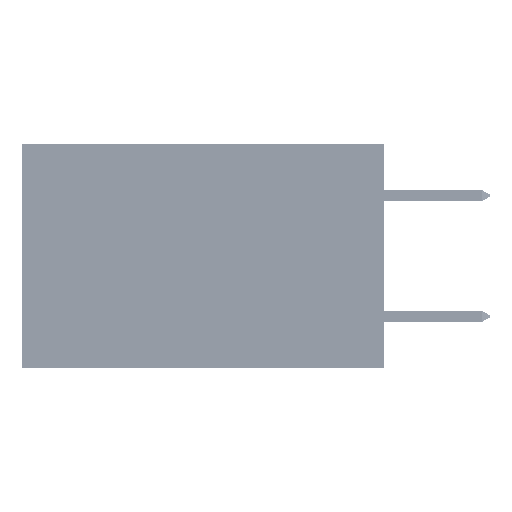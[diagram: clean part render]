
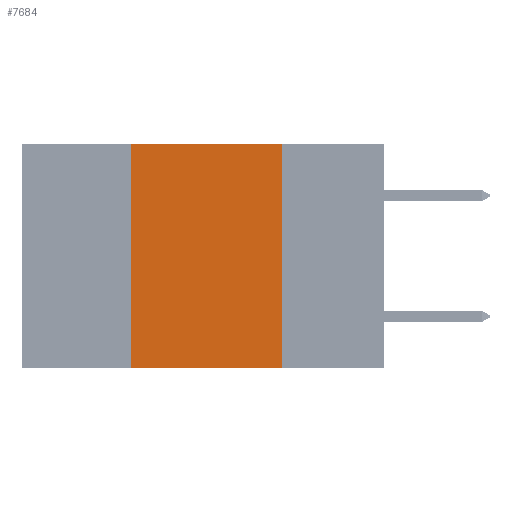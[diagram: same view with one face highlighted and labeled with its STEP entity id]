
A CAD part, left-side view. The second image highlights one B-rep face of the part: STEP entity #7684.
In plain terms, the highlighted planar face has unit normal (-1, 0, 0).
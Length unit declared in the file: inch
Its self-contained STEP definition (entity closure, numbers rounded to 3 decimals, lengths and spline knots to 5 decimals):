
#2695 = EDGE_LOOP ( 'NONE', ( #38751, #36651, #32935, #32762 ) ) ;
#6746 = EDGE_CURVE ( 'NONE', #7051, #33183, #30985, .T. ) ;
#7051 = VERTEX_POINT ( 'NONE', #43044 ) ;
#7213 = CARTESIAN_POINT ( 'NONE',  ( 0., 0.17, -0.37 ) ) ;
#7396 = VERTEX_POINT ( 'NONE', #7213 ) ;
#7684 = ADVANCED_FACE ( 'NONE', ( #33970 ), #12927, .F. ) ;
#9868 = VECTOR ( 'NONE', #33888, 39.37008 ) ;
#10032 = VECTOR ( 'NONE', #12802, 39.37008 ) ;
#12802 = DIRECTION ( 'NONE',  ( 0., 0., -1. ) ) ;
#12927 = PLANE ( 'NONE',  #21436 ) ;
#16139 = CARTESIAN_POINT ( 'NONE',  ( 0., 0.17, 0. ) ) ;
#16588 = DIRECTION ( 'NONE',  ( 0., 0., -1. ) ) ;
#20619 = LINE ( 'NONE', #16139, #10032 ) ;
#21436 = AXIS2_PLACEMENT_3D ( 'NONE', #40287, #24396, #16588 ) ;
#21465 = CARTESIAN_POINT ( 'NONE',  ( 0., 0.17, 0. ) ) ;
#21506 = EDGE_CURVE ( 'NONE', #43716, #7396, #25130, .T. ) ;
#24396 = DIRECTION ( 'NONE',  ( 1., 0., 0. ) ) ;
#25130 = LINE ( 'NONE', #29397, #26310 ) ;
#25636 = LINE ( 'NONE', #34599, #39239 ) ;
#26310 = VECTOR ( 'NONE', #29555, 39.37008 ) ;
#29397 = CARTESIAN_POINT ( 'NONE',  ( 0., 0.6, -0.37 ) ) ;
#29547 = CARTESIAN_POINT ( 'NONE',  ( 0., 0.6, 0. ) ) ;
#29555 = DIRECTION ( 'NONE',  ( 0., -1., 0. ) ) ;
#30985 = LINE ( 'NONE', #29547, #9868 ) ;
#32762 = ORIENTED_EDGE ( 'NONE', *, *, #21506, .T. ) ;
#32935 = ORIENTED_EDGE ( 'NONE', *, *, #47032, .F. ) ;
#33183 = VERTEX_POINT ( 'NONE', #21465 ) ;
#33888 = DIRECTION ( 'NONE',  ( 0., -1., 0. ) ) ;
#33970 = FACE_OUTER_BOUND ( 'NONE', #2695, .T. ) ;
#34599 = CARTESIAN_POINT ( 'NONE',  ( 0., 0.42, 0. ) ) ;
#34834 = CARTESIAN_POINT ( 'NONE',  ( 0., 0.42, -0.37 ) ) ;
#36651 = ORIENTED_EDGE ( 'NONE', *, *, #6746, .F. ) ;
#38751 = ORIENTED_EDGE ( 'NONE', *, *, #48564, .F. ) ;
#39239 = VECTOR ( 'NONE', #50597, 39.37008 ) ;
#40287 = CARTESIAN_POINT ( 'NONE',  ( 0., 0.6, 0. ) ) ;
#43044 = CARTESIAN_POINT ( 'NONE',  ( 0., 0.42, 0. ) ) ;
#43716 = VERTEX_POINT ( 'NONE', #34834 ) ;
#47032 = EDGE_CURVE ( 'NONE', #43716, #7051, #25636, .T. ) ;
#48564 = EDGE_CURVE ( 'NONE', #33183, #7396, #20619, .T. ) ;
#50597 = DIRECTION ( 'NONE',  ( 0., 0., 1. ) ) ;
